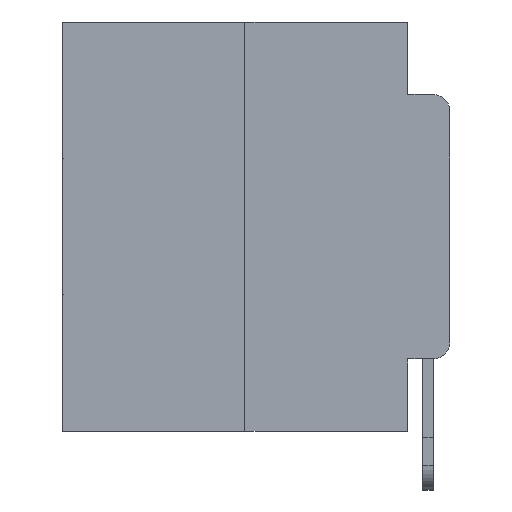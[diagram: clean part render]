
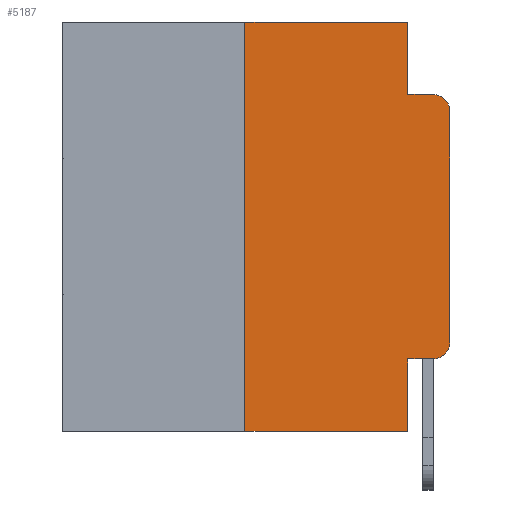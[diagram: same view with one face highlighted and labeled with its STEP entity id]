
A CAD part, left-side view. The second image highlights one B-rep face of the part: STEP entity #5187.
In plain terms, the highlighted planar face has unit normal (-1, 0, 0).
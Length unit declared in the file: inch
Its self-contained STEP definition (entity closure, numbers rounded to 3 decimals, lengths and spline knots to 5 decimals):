
#123 = ORIENTED_EDGE ( 'NONE', *, *, #7511, .T. ) ;
#359 = ORIENTED_EDGE ( 'NONE', *, *, #7560, .T. ) ;
#367 = CARTESIAN_POINT ( 'NONE',  ( 0., 0., -0.3915 ) ) ;
#721 = EDGE_CURVE ( 'NONE', #863, #24055, #4261, .T. ) ;
#863 = VERTEX_POINT ( 'NONE', #367 ) ;
#1386 = LINE ( 'NONE', #7267, #18603 ) ;
#1469 = ORIENTED_EDGE ( 'NONE', *, *, #721, .T. ) ;
#1847 = VECTOR ( 'NONE', #26750, 39.37008 ) ;
#1982 = DIRECTION ( 'NONE',  ( 0., 0., -1. ) ) ;
#2491 = ORIENTED_EDGE ( 'NONE', *, *, #19358, .F. ) ;
#2940 = EDGE_CURVE ( 'NONE', #24759, #863, #20039, .T. ) ;
#3143 = ORIENTED_EDGE ( 'NONE', *, *, #10518, .F. ) ;
#3634 = VECTOR ( 'NONE', #10192, 39.37008 ) ;
#3723 = CARTESIAN_POINT ( 'NONE',  ( 0., 0.25, 0. ) ) ;
#3964 = DIRECTION ( 'NONE',  ( 0., -1., 0. ) ) ;
#4261 = LINE ( 'NONE', #4400, #26851 ) ;
#4400 = CARTESIAN_POINT ( 'NONE',  ( 0., 0., 0. ) ) ;
#5187 = ADVANCED_FACE ( 'NONE', ( #16568 ), #7502, .F. ) ;
#5308 = DIRECTION ( 'NONE',  ( 1., 0., 0. ) ) ;
#6278 = VERTEX_POINT ( 'NONE', #20669 ) ;
#6704 = ORIENTED_EDGE ( 'NONE', *, *, #9033, .F. ) ;
#6706 = CARTESIAN_POINT ( 'NONE',  ( 0., 0.02, -0.3915 ) ) ;
#7205 = ORIENTED_EDGE ( 'NONE', *, *, #23642, .F. ) ;
#7267 = CARTESIAN_POINT ( 'NONE',  ( 0., 0.051, 0. ) ) ;
#7340 = ORIENTED_EDGE ( 'NONE', *, *, #25043, .T. ) ;
#7502 = PLANE ( 'NONE',  #10496 ) ;
#7511 = EDGE_CURVE ( 'NONE', #10048, #24759, #13202, .T. ) ;
#7560 = EDGE_CURVE ( 'NONE', #19311, #21172, #27638, .T. ) ;
#7799 = CARTESIAN_POINT ( 'NONE',  ( 0., 0.02, -0.4115 ) ) ;
#8379 = AXIS2_PLACEMENT_3D ( 'NONE', #6706, #22087, #9007 ) ;
#8545 = DIRECTION ( 'NONE',  ( 0., -1., 0. ) ) ;
#8980 = DIRECTION ( 'NONE',  ( 0., 0., 1. ) ) ;
#9007 = DIRECTION ( 'NONE',  ( 0., 0., -1. ) ) ;
#9033 = EDGE_CURVE ( 'NONE', #10048, #21172, #19984, .T. ) ;
#9457 = ORIENTED_EDGE ( 'NONE', *, *, #2940, .T. ) ;
#10000 = VERTEX_POINT ( 'NONE', #11516 ) ;
#10048 = VERTEX_POINT ( 'NONE', #11608 ) ;
#10189 = VECTOR ( 'NONE', #27839, 39.37008 ) ;
#10192 = DIRECTION ( 'NONE',  ( 0., 0., -1. ) ) ;
#10496 = AXIS2_PLACEMENT_3D ( 'NONE', #27058, #5308, #20787 ) ;
#10501 = CARTESIAN_POINT ( 'NONE',  ( 0., 0.051, -0.0885 ) ) ;
#10518 = EDGE_CURVE ( 'NONE', #19311, #24898, #25300, .T. ) ;
#10645 = LINE ( 'NONE', #15156, #15891 ) ;
#10862 = LINE ( 'NONE', #10501, #10189 ) ;
#10979 = DIRECTION ( 'NONE',  ( 0., -1., 0. ) ) ;
#11516 = CARTESIAN_POINT ( 'NONE',  ( 0., 0.02, -0.0885 ) ) ;
#11608 = CARTESIAN_POINT ( 'NONE',  ( 0., 0.051, -0.4115 ) ) ;
#11625 = EDGE_LOOP ( 'NONE', ( #1469, #7340, #7205, #2491, #21145, #3143, #359, #6704, #123, #9457 ) ) ;
#11960 = EDGE_CURVE ( 'NONE', #24898, #6278, #10645, .T. ) ;
#12298 = CARTESIAN_POINT ( 'NONE',  ( 0., 0.051, -0.0885 ) ) ;
#12890 = CIRCLE ( 'NONE', #27386, 0.02 ) ;
#13202 = LINE ( 'NONE', #27965, #25318 ) ;
#13634 = CARTESIAN_POINT ( 'NONE',  ( 0., 0.051, -0.5 ) ) ;
#15156 = CARTESIAN_POINT ( 'NONE',  ( 0., 0.473, 0. ) ) ;
#15495 = DIRECTION ( 'NONE',  ( -1., 0., 0. ) ) ;
#15891 = VECTOR ( 'NONE', #3964, 39.37008 ) ;
#16366 = VECTOR ( 'NONE', #10979, 39.37008 ) ;
#16568 = FACE_OUTER_BOUND ( 'NONE', #11625, .T. ) ;
#18117 = CARTESIAN_POINT ( 'NONE',  ( 0., 0.25, -0.5 ) ) ;
#18317 = DIRECTION ( 'NONE',  ( 0., 0., -1. ) ) ;
#18603 = VECTOR ( 'NONE', #18317, 39.37008 ) ;
#19311 = VERTEX_POINT ( 'NONE', #18117 ) ;
#19358 = EDGE_CURVE ( 'NONE', #6278, #24789, #1386, .T. ) ;
#19984 = LINE ( 'NONE', #23227, #3634 ) ;
#20039 = CIRCLE ( 'NONE', #8379, 0.02 ) ;
#20543 = CARTESIAN_POINT ( 'NONE',  ( 0., 0., -0.1085 ) ) ;
#20669 = CARTESIAN_POINT ( 'NONE',  ( 0., 0.051, 0. ) ) ;
#20787 = DIRECTION ( 'NONE',  ( 0., 0., -1. ) ) ;
#21145 = ORIENTED_EDGE ( 'NONE', *, *, #11960, .F. ) ;
#21172 = VERTEX_POINT ( 'NONE', #13634 ) ;
#22087 = DIRECTION ( 'NONE',  ( -1., 0., 0. ) ) ;
#23227 = CARTESIAN_POINT ( 'NONE',  ( 0., 0.051, 0. ) ) ;
#23642 = EDGE_CURVE ( 'NONE', #24789, #10000, #10862, .T. ) ;
#24055 = VERTEX_POINT ( 'NONE', #20543 ) ;
#24633 = CARTESIAN_POINT ( 'NONE',  ( 0., 0.25, 0. ) ) ;
#24759 = VERTEX_POINT ( 'NONE', #7799 ) ;
#24789 = VERTEX_POINT ( 'NONE', #12298 ) ;
#24898 = VERTEX_POINT ( 'NONE', #3723 ) ;
#25043 = EDGE_CURVE ( 'NONE', #24055, #10000, #12890, .T. ) ;
#25300 = LINE ( 'NONE', #24633, #1847 ) ;
#25318 = VECTOR ( 'NONE', #8545, 39.37008 ) ;
#26750 = DIRECTION ( 'NONE',  ( 0., 0., 1. ) ) ;
#26851 = VECTOR ( 'NONE', #8980, 39.37008 ) ;
#27058 = CARTESIAN_POINT ( 'NONE',  ( 0., 0.473, 0. ) ) ;
#27386 = AXIS2_PLACEMENT_3D ( 'NONE', #28267, #15495, #1982 ) ;
#27638 = LINE ( 'NONE', #28136, #16366 ) ;
#27839 = DIRECTION ( 'NONE',  ( 0., -1., 0. ) ) ;
#27965 = CARTESIAN_POINT ( 'NONE',  ( 0., 0.051, -0.4115 ) ) ;
#28136 = CARTESIAN_POINT ( 'NONE',  ( 0., 0.473, -0.5 ) ) ;
#28267 = CARTESIAN_POINT ( 'NONE',  ( 0., 0.02, -0.1085 ) ) ;
